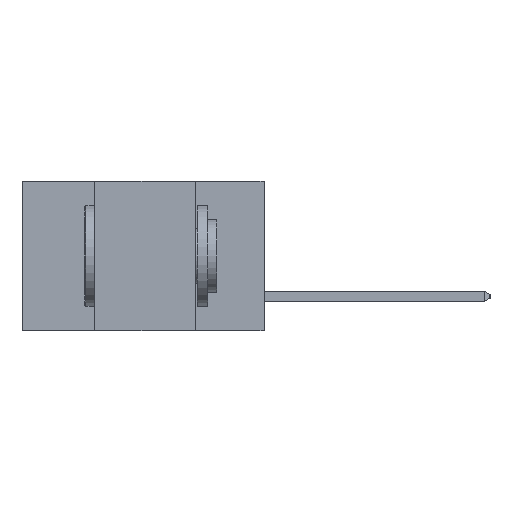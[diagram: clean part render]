
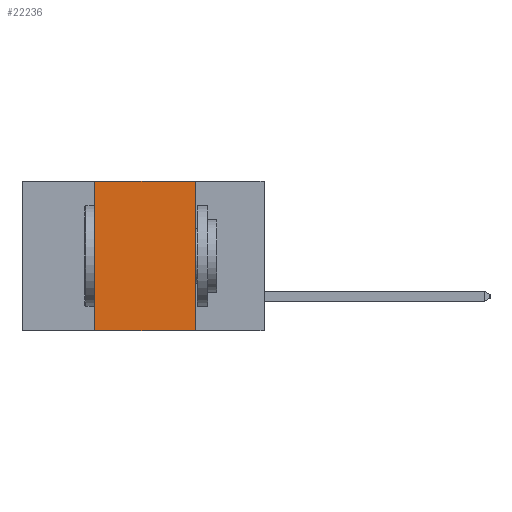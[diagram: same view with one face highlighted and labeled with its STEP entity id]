
A CAD part, left-side view. The second image highlights one B-rep face of the part: STEP entity #22236.
In plain terms, the highlighted planar face has unit normal (-1, 0, 0).
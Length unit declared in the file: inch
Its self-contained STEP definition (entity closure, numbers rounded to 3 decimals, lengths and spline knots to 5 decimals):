
#1256 = DIRECTION ( 'NONE',  ( 0., 0., -1. ) ) ;
#1578 = CARTESIAN_POINT ( 'NONE',  ( 0., 0.42, 0. ) ) ;
#1962 = EDGE_CURVE ( 'NONE', #2272, #15185, #22510, .T. ) ;
#2128 = DIRECTION ( 'NONE',  ( 0., -1., 0. ) ) ;
#2272 = VERTEX_POINT ( 'NONE', #13494 ) ;
#5780 = ORIENTED_EDGE ( 'NONE', *, *, #1962, .F. ) ;
#6079 = ORIENTED_EDGE ( 'NONE', *, *, #10060, .F. ) ;
#6591 = VERTEX_POINT ( 'NONE', #25326 ) ;
#6684 = PLANE ( 'NONE',  #17584 ) ;
#7398 = EDGE_LOOP ( 'NONE', ( #9836, #6079, #5780, #15642 ) ) ;
#7590 = VECTOR ( 'NONE', #8484, 39.37008 ) ;
#8484 = DIRECTION ( 'NONE',  ( 0., 0., 1. ) ) ;
#8706 = DIRECTION ( 'NONE',  ( 0., 0., -1. ) ) ;
#9836 = ORIENTED_EDGE ( 'NONE', *, *, #16597, .F. ) ;
#10036 = LINE ( 'NONE', #24806, #17943 ) ;
#10060 = EDGE_CURVE ( 'NONE', #15185, #6591, #17082, .T. ) ;
#11750 = DIRECTION ( 'NONE',  ( 0., -1., 0. ) ) ;
#12138 = FACE_OUTER_BOUND ( 'NONE', #7398, .T. ) ;
#12986 = CARTESIAN_POINT ( 'NONE',  ( 0., 0.17, -0.37 ) ) ;
#13494 = CARTESIAN_POINT ( 'NONE',  ( 0., 0.42, -0.37 ) ) ;
#14287 = CARTESIAN_POINT ( 'NONE',  ( 0., 0.6, 0. ) ) ;
#15185 = VERTEX_POINT ( 'NONE', #1578 ) ;
#15642 = ORIENTED_EDGE ( 'NONE', *, *, #24818, .T. ) ;
#16464 = VECTOR ( 'NONE', #11750, 39.37008 ) ;
#16597 = EDGE_CURVE ( 'NONE', #6591, #24209, #10036, .T. ) ;
#17082 = LINE ( 'NONE', #14287, #16464 ) ;
#17584 = AXIS2_PLACEMENT_3D ( 'NONE', #22199, #20320, #8706 ) ;
#17943 = VECTOR ( 'NONE', #1256, 39.37008 ) ;
#19143 = LINE ( 'NONE', #23687, #23690 ) ;
#20320 = DIRECTION ( 'NONE',  ( 1., 0., 0. ) ) ;
#20359 = CARTESIAN_POINT ( 'NONE',  ( 0., 0.42, -0.37 ) ) ;
#22199 = CARTESIAN_POINT ( 'NONE',  ( 0., 0.6, 0. ) ) ;
#22236 = ADVANCED_FACE ( 'NONE', ( #12138 ), #6684, .F. ) ;
#22510 = LINE ( 'NONE', #20359, #7590 ) ;
#23687 = CARTESIAN_POINT ( 'NONE',  ( 0., 0.6, -0.37 ) ) ;
#23690 = VECTOR ( 'NONE', #2128, 39.37008 ) ;
#24209 = VERTEX_POINT ( 'NONE', #12986 ) ;
#24806 = CARTESIAN_POINT ( 'NONE',  ( 0., 0.17, -0.37 ) ) ;
#24818 = EDGE_CURVE ( 'NONE', #2272, #24209, #19143, .T. ) ;
#25326 = CARTESIAN_POINT ( 'NONE',  ( 0., 0.17, 0. ) ) ;
